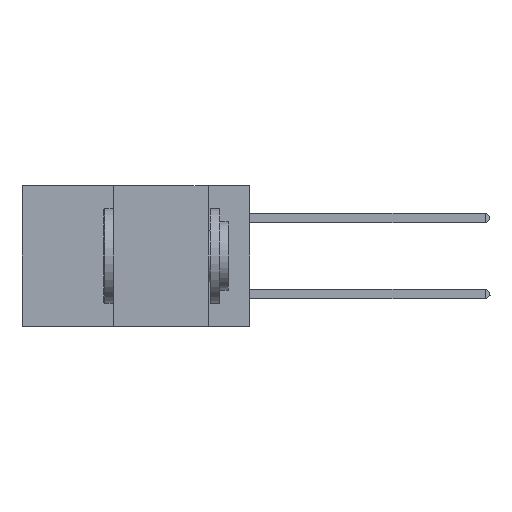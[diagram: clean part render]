
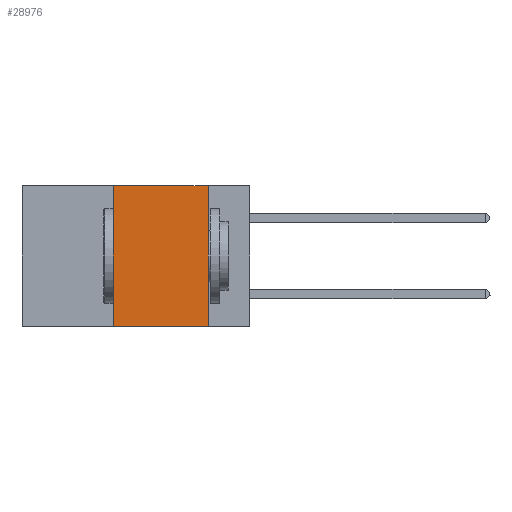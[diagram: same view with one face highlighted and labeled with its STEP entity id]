
A CAD part, left-side view. The second image highlights one B-rep face of the part: STEP entity #28976.
In plain terms, the highlighted planar face has unit normal (-1, 0, 0).
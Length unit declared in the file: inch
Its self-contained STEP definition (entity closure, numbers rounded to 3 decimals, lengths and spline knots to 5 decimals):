
#377 = EDGE_CURVE ( 'NONE', #5920, #1680, #13283, .T. ) ;
#447 = LINE ( 'NONE', #8875, #8309 ) ;
#1147 = VERTEX_POINT ( 'NONE', #29462 ) ;
#1680 = VERTEX_POINT ( 'NONE', #28164 ) ;
#1780 = LINE ( 'NONE', #8475, #22680 ) ;
#3752 = CARTESIAN_POINT ( 'NONE',  ( 0., 0.11, 0. ) ) ;
#5565 = DIRECTION ( 'NONE',  ( 0., 0., -1. ) ) ;
#5920 = VERTEX_POINT ( 'NONE', #17961 ) ;
#7877 = PLANE ( 'NONE',  #14215 ) ;
#7962 = EDGE_CURVE ( 'NONE', #1147, #1680, #21313, .T. ) ;
#8309 = VECTOR ( 'NONE', #13530, 39.37008 ) ;
#8475 = CARTESIAN_POINT ( 'NONE',  ( 0., 0.6, 0. ) ) ;
#8875 = CARTESIAN_POINT ( 'NONE',  ( 0., 0.36, 0. ) ) ;
#9902 = ORIENTED_EDGE ( 'NONE', *, *, #18767, .F. ) ;
#12444 = CARTESIAN_POINT ( 'NONE',  ( 0., 0.6, 0. ) ) ;
#13220 = DIRECTION ( 'NONE',  ( 0., 0., -1. ) ) ;
#13273 = FACE_OUTER_BOUND ( 'NONE', #16441, .T. ) ;
#13283 = LINE ( 'NONE', #3752, #27354 ) ;
#13530 = DIRECTION ( 'NONE',  ( 0., 0., 1. ) ) ;
#13631 = DIRECTION ( 'NONE',  ( 0., -1., 0. ) ) ;
#14215 = AXIS2_PLACEMENT_3D ( 'NONE', #12444, #28781, #5565 ) ;
#14897 = CARTESIAN_POINT ( 'NONE',  ( 0., 0.36, 0. ) ) ;
#15189 = VERTEX_POINT ( 'NONE', #14897 ) ;
#16441 = EDGE_LOOP ( 'NONE', ( #20282, #9902, #23888, #22953 ) ) ;
#17298 = EDGE_CURVE ( 'NONE', #1147, #15189, #447, .T. ) ;
#17961 = CARTESIAN_POINT ( 'NONE',  ( 0., 0.11, 0. ) ) ;
#18628 = CARTESIAN_POINT ( 'NONE',  ( 0., 0.6, -0.37 ) ) ;
#18767 = EDGE_CURVE ( 'NONE', #15189, #5920, #1780, .T. ) ;
#20282 = ORIENTED_EDGE ( 'NONE', *, *, #377, .F. ) ;
#21153 = DIRECTION ( 'NONE',  ( 0., -1., 0. ) ) ;
#21313 = LINE ( 'NONE', #18628, #24188 ) ;
#22680 = VECTOR ( 'NONE', #13631, 39.37008 ) ;
#22953 = ORIENTED_EDGE ( 'NONE', *, *, #7962, .T. ) ;
#23888 = ORIENTED_EDGE ( 'NONE', *, *, #17298, .F. ) ;
#24188 = VECTOR ( 'NONE', #21153, 39.37008 ) ;
#27354 = VECTOR ( 'NONE', #13220, 39.37008 ) ;
#28164 = CARTESIAN_POINT ( 'NONE',  ( 0., 0.11, -0.37 ) ) ;
#28781 = DIRECTION ( 'NONE',  ( 1., 0., 0. ) ) ;
#28976 = ADVANCED_FACE ( 'NONE', ( #13273 ), #7877, .F. ) ;
#29462 = CARTESIAN_POINT ( 'NONE',  ( 0., 0.36, -0.37 ) ) ;
